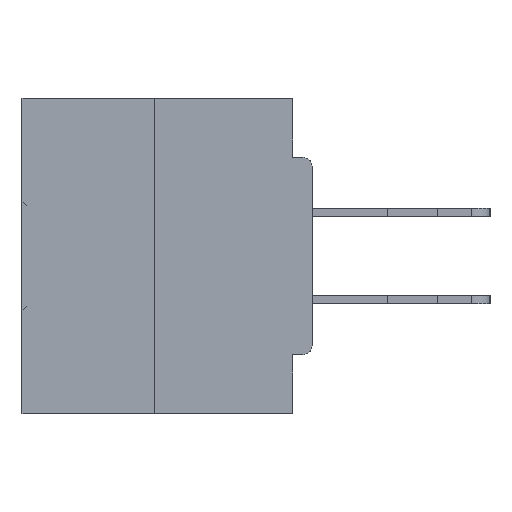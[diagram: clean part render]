
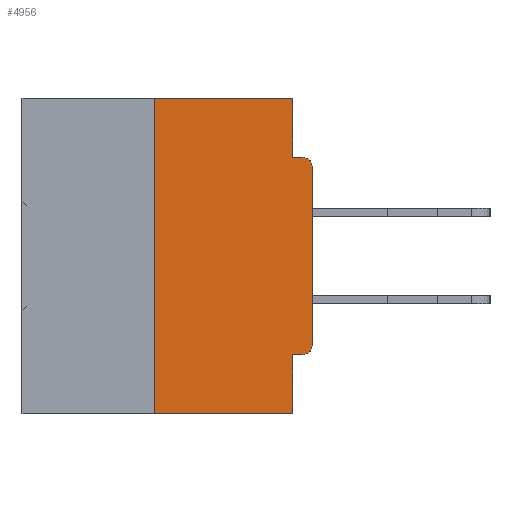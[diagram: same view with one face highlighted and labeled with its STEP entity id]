
A CAD part, left-side view. The second image highlights one B-rep face of the part: STEP entity #4956.
In plain terms, the highlighted planar face has unit normal (-1, 0, 0).
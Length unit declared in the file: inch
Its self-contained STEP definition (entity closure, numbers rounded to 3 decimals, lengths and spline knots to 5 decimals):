
#695 = CARTESIAN_POINT ( 'NONE',  ( 0., 0.031, 0. ) ) ;
#986 = ORIENTED_EDGE ( 'NONE', *, *, #12291, .T. ) ;
#1126 = ORIENTED_EDGE ( 'NONE', *, *, #9623, .F. ) ;
#1755 = LINE ( 'NONE', #14647, #13591 ) ;
#2529 = CARTESIAN_POINT ( 'NONE',  ( 0., 0.031, -0.5 ) ) ;
#2626 = ORIENTED_EDGE ( 'NONE', *, *, #25565, .F. ) ;
#3892 = CARTESIAN_POINT ( 'NONE',  ( 0., 0.46, -0.5 ) ) ;
#4706 = VERTEX_POINT ( 'NONE', #33566 ) ;
#4956 = ADVANCED_FACE ( 'NONE', ( #26622 ), #37680, .F. ) ;
#5035 = EDGE_CURVE ( 'NONE', #11052, #40494, #35077, .T. ) ;
#5421 = VECTOR ( 'NONE', #42862, 39.37008 ) ;
#5821 = AXIS2_PLACEMENT_3D ( 'NONE', #26430, #9026, #44500 ) ;
#6342 = EDGE_CURVE ( 'NONE', #34708, #21644, #13431, .T. ) ;
#7008 = ORIENTED_EDGE ( 'NONE', *, *, #40202, .F. ) ;
#7218 = LINE ( 'NONE', #28211, #36669 ) ;
#7644 = AXIS2_PLACEMENT_3D ( 'NONE', #43208, #14215, #32581 ) ;
#8091 = CARTESIAN_POINT ( 'NONE',  ( 0., 0., -0.3915 ) ) ;
#8435 = ORIENTED_EDGE ( 'NONE', *, *, #9954, .F. ) ;
#9026 = DIRECTION ( 'NONE',  ( 1., 0., 0. ) ) ;
#9281 = LINE ( 'NONE', #695, #14344 ) ;
#9623 = EDGE_CURVE ( 'NONE', #23944, #16630, #9281, .T. ) ;
#9954 = EDGE_CURVE ( 'NONE', #4706, #23944, #7218, .T. ) ;
#10983 = DIRECTION ( 'NONE',  ( 0., -1., 0. ) ) ;
#11052 = VERTEX_POINT ( 'NONE', #40424 ) ;
#12161 = DIRECTION ( 'NONE',  ( 0., 0., 1. ) ) ;
#12216 = LINE ( 'NONE', #24970, #5421 ) ;
#12291 = EDGE_CURVE ( 'NONE', #21644, #22033, #42663, .T. ) ;
#12925 = EDGE_CURVE ( 'NONE', #16737, #40494, #23908, .T. ) ;
#13215 = CARTESIAN_POINT ( 'NONE',  ( 0., 0., -0.1085 ) ) ;
#13431 = LINE ( 'NONE', #42315, #32138 ) ;
#13591 = VECTOR ( 'NONE', #39862, 39.37008 ) ;
#14215 = DIRECTION ( 'NONE',  ( -1., 0., 0. ) ) ;
#14344 = VECTOR ( 'NONE', #26754, 39.37008 ) ;
#14457 = ORIENTED_EDGE ( 'NONE', *, *, #6342, .T. ) ;
#14628 = CARTESIAN_POINT ( 'NONE',  ( 0., 0.015, -0.3915 ) ) ;
#14647 = CARTESIAN_POINT ( 'NONE',  ( 0., 0., -0.0935 ) ) ;
#14791 = DIRECTION ( 'NONE',  ( 0., 0., -1. ) ) ;
#14797 = EDGE_CURVE ( 'NONE', #41694, #34708, #38518, .T. ) ;
#15329 = LINE ( 'NONE', #19924, #46520 ) ;
#15836 = VECTOR ( 'NONE', #20538, 39.37008 ) ;
#16630 = VERTEX_POINT ( 'NONE', #46073 ) ;
#16737 = VERTEX_POINT ( 'NONE', #32399 ) ;
#19544 = CARTESIAN_POINT ( 'NONE',  ( 0., 0.031, -0.5 ) ) ;
#19728 = ORIENTED_EDGE ( 'NONE', *, *, #5035, .F. ) ;
#19924 = CARTESIAN_POINT ( 'NONE',  ( 0., 0.25, 0. ) ) ;
#20538 = DIRECTION ( 'NONE',  ( 0., 0., -1. ) ) ;
#21064 = DIRECTION ( 'NONE',  ( 0., 0., 1. ) ) ;
#21435 = DIRECTION ( 'NONE',  ( 0., -1., 0. ) ) ;
#21644 = VERTEX_POINT ( 'NONE', #13215 ) ;
#21929 = DIRECTION ( 'NONE',  ( -1., 0., 0. ) ) ;
#22033 = VERTEX_POINT ( 'NONE', #43951 ) ;
#23771 = EDGE_LOOP ( 'NONE', ( #8435, #2626, #28919, #19728, #7008, #25935, #14457, #986, #43230, #1126 ) ) ;
#23908 = LINE ( 'NONE', #3892, #34680 ) ;
#23944 = VERTEX_POINT ( 'NONE', #33168 ) ;
#24970 = CARTESIAN_POINT ( 'NONE',  ( 0., 0., -0.4065 ) ) ;
#25565 = EDGE_CURVE ( 'NONE', #16737, #4706, #15329, .T. ) ;
#25928 = EDGE_CURVE ( 'NONE', #16630, #22033, #1755, .T. ) ;
#25935 = ORIENTED_EDGE ( 'NONE', *, *, #14797, .T. ) ;
#25945 = AXIS2_PLACEMENT_3D ( 'NONE', #14628, #21929, #14791 ) ;
#26412 = CARTESIAN_POINT ( 'NONE',  ( 0., 0.015, -0.4065 ) ) ;
#26430 = CARTESIAN_POINT ( 'NONE',  ( 0., 0.46, 0. ) ) ;
#26622 = FACE_OUTER_BOUND ( 'NONE', #23771, .T. ) ;
#26754 = DIRECTION ( 'NONE',  ( 0., 0., -1. ) ) ;
#28211 = CARTESIAN_POINT ( 'NONE',  ( 0., 0.46, 0. ) ) ;
#28919 = ORIENTED_EDGE ( 'NONE', *, *, #12925, .T. ) ;
#32138 = VECTOR ( 'NONE', #21064, 39.37008 ) ;
#32399 = CARTESIAN_POINT ( 'NONE',  ( 0., 0.25, -0.5 ) ) ;
#32581 = DIRECTION ( 'NONE',  ( 0., 0., -1. ) ) ;
#33168 = CARTESIAN_POINT ( 'NONE',  ( 0., 0.031, 0. ) ) ;
#33566 = CARTESIAN_POINT ( 'NONE',  ( 0., 0.25, 0. ) ) ;
#34680 = VECTOR ( 'NONE', #10983, 39.37008 ) ;
#34708 = VERTEX_POINT ( 'NONE', #8091 ) ;
#35077 = LINE ( 'NONE', #2529, #15836 ) ;
#36669 = VECTOR ( 'NONE', #21435, 39.37008 ) ;
#37680 = PLANE ( 'NONE',  #5821 ) ;
#38518 = CIRCLE ( 'NONE', #25945, 0.015 ) ;
#39862 = DIRECTION ( 'NONE',  ( 0., -1., 0. ) ) ;
#40202 = EDGE_CURVE ( 'NONE', #41694, #11052, #12216, .T. ) ;
#40424 = CARTESIAN_POINT ( 'NONE',  ( 0., 0.031, -0.4065 ) ) ;
#40494 = VERTEX_POINT ( 'NONE', #19544 ) ;
#41694 = VERTEX_POINT ( 'NONE', #26412 ) ;
#42315 = CARTESIAN_POINT ( 'NONE',  ( 0., 0., 0. ) ) ;
#42663 = CIRCLE ( 'NONE', #7644, 0.015 ) ;
#42862 = DIRECTION ( 'NONE',  ( 0., 1., 0. ) ) ;
#43208 = CARTESIAN_POINT ( 'NONE',  ( 0., 0.015, -0.1085 ) ) ;
#43230 = ORIENTED_EDGE ( 'NONE', *, *, #25928, .F. ) ;
#43951 = CARTESIAN_POINT ( 'NONE',  ( 0., 0.015, -0.0935 ) ) ;
#44500 = DIRECTION ( 'NONE',  ( 0., 0., -1. ) ) ;
#46073 = CARTESIAN_POINT ( 'NONE',  ( 0., 0.031, -0.0935 ) ) ;
#46520 = VECTOR ( 'NONE', #12161, 39.37008 ) ;
